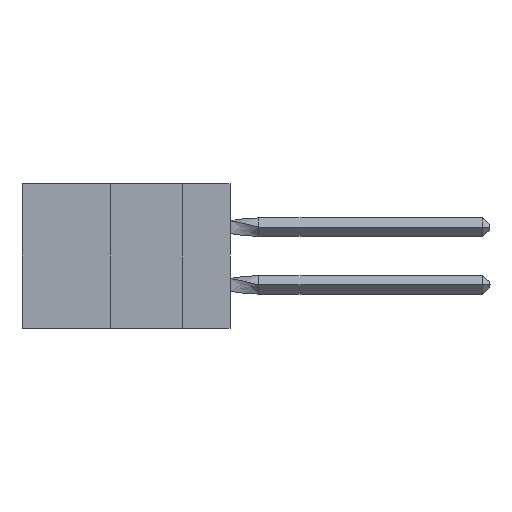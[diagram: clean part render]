
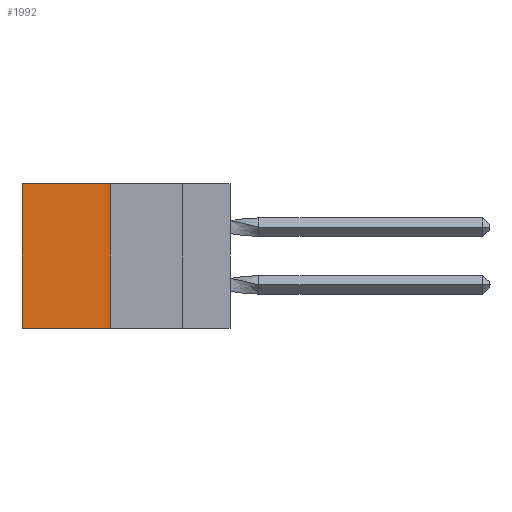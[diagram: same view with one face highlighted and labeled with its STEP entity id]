
A CAD part, left-side view. The second image highlights one B-rep face of the part: STEP entity #1992.
In plain terms, the highlighted planar face has unit normal (-1, 0, 0).
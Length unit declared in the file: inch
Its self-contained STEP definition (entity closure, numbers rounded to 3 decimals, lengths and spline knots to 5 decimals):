
#362 = DIRECTION ( 'NONE',  ( 0., 0., -1. ) ) ;
#1992 = ADVANCED_FACE ( 'NONE', ( #14463 ), #11559, .F. ) ;
#2345 = LINE ( 'NONE', #13776, #16132 ) ;
#2578 = ORIENTED_EDGE ( 'NONE', *, *, #15667, .T. ) ;
#2596 = LINE ( 'NONE', #9061, #14400 ) ;
#3232 = EDGE_CURVE ( 'NONE', #5202, #15662, #11075, .T. ) ;
#3275 = DIRECTION ( 'NONE',  ( 0., 0., -1. ) ) ;
#3411 = CARTESIAN_POINT ( 'NONE',  ( 0.305, 0.413, -0.5 ) ) ;
#3742 = VECTOR ( 'NONE', #3275, 39.37008 ) ;
#4059 = CARTESIAN_POINT ( 'NONE',  ( 0.305, 0.72, -0.5 ) ) ;
#4155 = DIRECTION ( 'NONE',  ( 1., 0., 0. ) ) ;
#5202 = VERTEX_POINT ( 'NONE', #3411 ) ;
#5507 = VERTEX_POINT ( 'NONE', #8303 ) ;
#6228 = DIRECTION ( 'NONE',  ( 0., 1., 0. ) ) ;
#7764 = VECTOR ( 'NONE', #11719, 39.37008 ) ;
#8303 = CARTESIAN_POINT ( 'NONE',  ( 0.305, 0.72, 0. ) ) ;
#8568 = EDGE_CURVE ( 'NONE', #10832, #5507, #2345, .T. ) ;
#8727 = ORIENTED_EDGE ( 'NONE', *, *, #8892, .F. ) ;
#8892 = EDGE_CURVE ( 'NONE', #10832, #5202, #11606, .T. ) ;
#9061 = CARTESIAN_POINT ( 'NONE',  ( 0.305, 0.72, -0.5 ) ) ;
#9088 = CARTESIAN_POINT ( 'NONE',  ( 0.305, 0.413, -0.5 ) ) ;
#9683 = CARTESIAN_POINT ( 'NONE',  ( 0.305, 0.413, -0.5 ) ) ;
#10695 = ORIENTED_EDGE ( 'NONE', *, *, #3232, .F. ) ;
#10832 = VERTEX_POINT ( 'NONE', #12517 ) ;
#11075 = LINE ( 'NONE', #9088, #7764 ) ;
#11559 = PLANE ( 'NONE',  #15170 ) ;
#11606 = LINE ( 'NONE', #9683, #3742 ) ;
#11623 = CARTESIAN_POINT ( 'NONE',  ( 0.305, 0.413, -0.5 ) ) ;
#11719 = DIRECTION ( 'NONE',  ( 0., 1., 0. ) ) ;
#11846 = ORIENTED_EDGE ( 'NONE', *, *, #8568, .T. ) ;
#12517 = CARTESIAN_POINT ( 'NONE',  ( 0.305, 0.413, 0. ) ) ;
#12852 = DIRECTION ( 'NONE',  ( 0., 0., -1. ) ) ;
#13776 = CARTESIAN_POINT ( 'NONE',  ( 0.305, 0.413, 0. ) ) ;
#14400 = VECTOR ( 'NONE', #12852, 39.37008 ) ;
#14463 = FACE_OUTER_BOUND ( 'NONE', #15158, .T. ) ;
#15158 = EDGE_LOOP ( 'NONE', ( #2578, #10695, #8727, #11846 ) ) ;
#15170 = AXIS2_PLACEMENT_3D ( 'NONE', #11623, #4155, #362 ) ;
#15662 = VERTEX_POINT ( 'NONE', #4059 ) ;
#15667 = EDGE_CURVE ( 'NONE', #5507, #15662, #2596, .T. ) ;
#16132 = VECTOR ( 'NONE', #6228, 39.37008 ) ;
